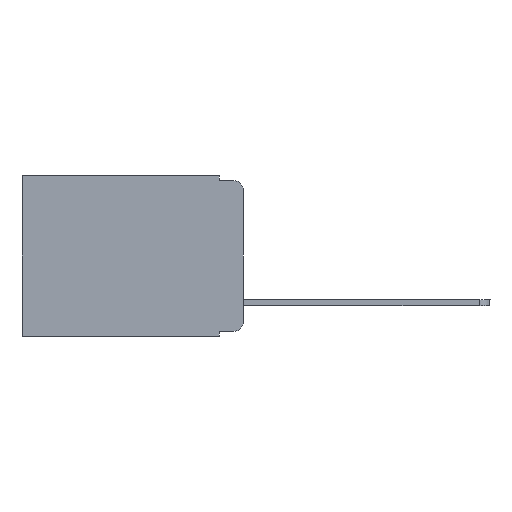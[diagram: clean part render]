
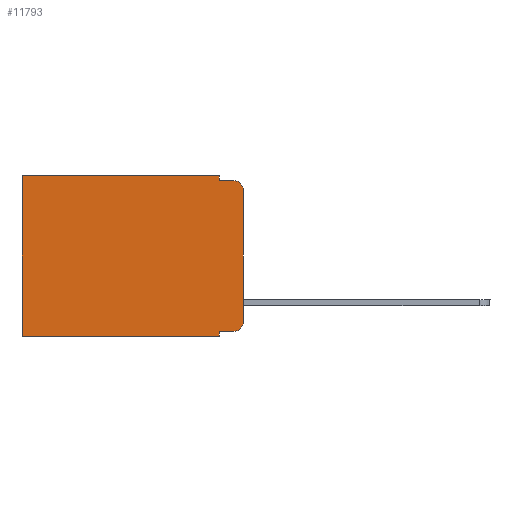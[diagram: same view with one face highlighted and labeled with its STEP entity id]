
A CAD part, left-side view. The second image highlights one B-rep face of the part: STEP entity #11793.
In plain terms, the highlighted planar face has unit normal (-1, 0, 0).
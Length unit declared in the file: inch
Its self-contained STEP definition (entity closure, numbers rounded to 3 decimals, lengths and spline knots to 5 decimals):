
#476 = VERTEX_POINT ( 'NONE', #9377 ) ;
#605 = EDGE_LOOP ( 'NONE', ( #9078, #6765, #993, #13070, #1900, #7192, #5269, #7069, #10858, #4568 ) ) ;
#840 = CARTESIAN_POINT ( 'NONE',  ( 0.298, 0.473, 0. ) ) ;
#993 = ORIENTED_EDGE ( 'NONE', *, *, #6296, .F. ) ;
#1261 = CARTESIAN_POINT ( 'NONE',  ( 0.298, 0.02, -0.03 ) ) ;
#1284 = DIRECTION ( 'NONE',  ( 0., 0., -1. ) ) ;
#1359 = CARTESIAN_POINT ( 'NONE',  ( 0.298, 0.473, -0.343 ) ) ;
#1796 = CARTESIAN_POINT ( 'NONE',  ( 0.298, 0., -0.03 ) ) ;
#1894 = LINE ( 'NONE', #2930, #6676 ) ;
#1900 = ORIENTED_EDGE ( 'NONE', *, *, #7040, .T. ) ;
#1941 = LINE ( 'NONE', #12450, #11049 ) ;
#2186 = PLANE ( 'NONE',  #11965 ) ;
#2492 = VERTEX_POINT ( 'NONE', #10042 ) ;
#2495 = CARTESIAN_POINT ( 'NONE',  ( 0.298, 0.02, -0.333 ) ) ;
#2696 = VECTOR ( 'NONE', #3556, 39.37008 ) ;
#2858 = VERTEX_POINT ( 'NONE', #13397 ) ;
#2930 = CARTESIAN_POINT ( 'NONE',  ( 0.298, 0.051, -0.333 ) ) ;
#3556 = DIRECTION ( 'NONE',  ( 0., 0., -1. ) ) ;
#3610 = DIRECTION ( 'NONE',  ( 0., 1., 0. ) ) ;
#3812 = CARTESIAN_POINT ( 'NONE',  ( 0.298, 0., 0. ) ) ;
#3837 = CARTESIAN_POINT ( 'NONE',  ( 0.298, 0.051, -0.343 ) ) ;
#3900 = DIRECTION ( 'NONE',  ( 0., -1., 0. ) ) ;
#3905 = EDGE_CURVE ( 'NONE', #4209, #2492, #10246, .T. ) ;
#4072 = CIRCLE ( 'NONE', #11988, 0.02 ) ;
#4209 = VERTEX_POINT ( 'NONE', #1796 ) ;
#4471 = DIRECTION ( 'NONE',  ( 1., 0., 0. ) ) ;
#4568 = ORIENTED_EDGE ( 'NONE', *, *, #6722, .T. ) ;
#4793 = CARTESIAN_POINT ( 'NONE',  ( 0.298, 0., -0.313 ) ) ;
#5070 = DIRECTION ( 'NONE',  ( 0., 0., -1. ) ) ;
#5269 = ORIENTED_EDGE ( 'NONE', *, *, #10959, .F. ) ;
#5420 = DIRECTION ( 'NONE',  ( 0., 0., -1. ) ) ;
#5440 = LINE ( 'NONE', #10599, #9110 ) ;
#6147 = VECTOR ( 'NONE', #5070, 39.37008 ) ;
#6296 = EDGE_CURVE ( 'NONE', #476, #2492, #5440, .T. ) ;
#6297 = AXIS2_PLACEMENT_3D ( 'NONE', #1261, #10580, #5420 ) ;
#6389 = DIRECTION ( 'NONE',  ( -1., 0., 0. ) ) ;
#6676 = VECTOR ( 'NONE', #3900, 39.37008 ) ;
#6722 = EDGE_CURVE ( 'NONE', #13594, #12317, #4072, .T. ) ;
#6765 = ORIENTED_EDGE ( 'NONE', *, *, #3905, .T. ) ;
#7040 = EDGE_CURVE ( 'NONE', #8321, #11954, #13282, .T. ) ;
#7058 = EDGE_CURVE ( 'NONE', #11954, #8721, #13421, .T. ) ;
#7069 = ORIENTED_EDGE ( 'NONE', *, *, #11130, .F. ) ;
#7123 = DIRECTION ( 'NONE',  ( 0., 0., -1. ) ) ;
#7192 = ORIENTED_EDGE ( 'NONE', *, *, #7058, .T. ) ;
#7750 = LINE ( 'NONE', #11960, #9729 ) ;
#8321 = VERTEX_POINT ( 'NONE', #10301 ) ;
#8598 = FACE_OUTER_BOUND ( 'NONE', #605, .T. ) ;
#8721 = VERTEX_POINT ( 'NONE', #1359 ) ;
#9078 = ORIENTED_EDGE ( 'NONE', *, *, #11810, .F. ) ;
#9110 = VECTOR ( 'NONE', #11783, 39.37008 ) ;
#9185 = CARTESIAN_POINT ( 'NONE',  ( 0.298, 0.051, 0. ) ) ;
#9193 = DIRECTION ( 'NONE',  ( 0., 1., 0. ) ) ;
#9377 = CARTESIAN_POINT ( 'NONE',  ( 0.298, 0.051, -0.01 ) ) ;
#9729 = VECTOR ( 'NONE', #3610, 39.37008 ) ;
#10042 = CARTESIAN_POINT ( 'NONE',  ( 0.298, 0.02, -0.01 ) ) ;
#10246 = CIRCLE ( 'NONE', #6297, 0.02 ) ;
#10301 = CARTESIAN_POINT ( 'NONE',  ( 0.298, 0.051, 0. ) ) ;
#10580 = DIRECTION ( 'NONE',  ( -1., 0., 0. ) ) ;
#10599 = CARTESIAN_POINT ( 'NONE',  ( 0.298, 0.051, -0.01 ) ) ;
#10739 = CARTESIAN_POINT ( 'NONE',  ( 0.298, 0., 0. ) ) ;
#10858 = ORIENTED_EDGE ( 'NONE', *, *, #12032, .T. ) ;
#10959 = EDGE_CURVE ( 'NONE', #11835, #8721, #7750, .T. ) ;
#11049 = VECTOR ( 'NONE', #7123, 39.37008 ) ;
#11071 = LINE ( 'NONE', #11207, #2696 ) ;
#11130 = EDGE_CURVE ( 'NONE', #2858, #11835, #1941, .T. ) ;
#11207 = CARTESIAN_POINT ( 'NONE',  ( 0.298, 0., 0. ) ) ;
#11245 = DIRECTION ( 'NONE',  ( 0., 0., -1. ) ) ;
#11353 = CARTESIAN_POINT ( 'NONE',  ( 0.298, 0.473, 0. ) ) ;
#11783 = DIRECTION ( 'NONE',  ( 0., -1., 0. ) ) ;
#11793 = ADVANCED_FACE ( 'NONE', ( #8598 ), #2186, .F. ) ;
#11810 = EDGE_CURVE ( 'NONE', #4209, #12317, #11071, .T. ) ;
#11835 = VERTEX_POINT ( 'NONE', #3837 ) ;
#11954 = VERTEX_POINT ( 'NONE', #11353 ) ;
#11960 = CARTESIAN_POINT ( 'NONE',  ( 0.298, 0., -0.343 ) ) ;
#11965 = AXIS2_PLACEMENT_3D ( 'NONE', #10739, #4471, #1284 ) ;
#11988 = AXIS2_PLACEMENT_3D ( 'NONE', #13586, #6389, #13646 ) ;
#12032 = EDGE_CURVE ( 'NONE', #2858, #13594, #1894, .T. ) ;
#12316 = VECTOR ( 'NONE', #9193, 39.37008 ) ;
#12317 = VERTEX_POINT ( 'NONE', #4793 ) ;
#12450 = CARTESIAN_POINT ( 'NONE',  ( 0.298, 0.051, 0. ) ) ;
#12583 = LINE ( 'NONE', #9185, #13532 ) ;
#12631 = EDGE_CURVE ( 'NONE', #8321, #476, #12583, .T. ) ;
#13070 = ORIENTED_EDGE ( 'NONE', *, *, #12631, .F. ) ;
#13282 = LINE ( 'NONE', #3812, #12316 ) ;
#13397 = CARTESIAN_POINT ( 'NONE',  ( 0.298, 0.051, -0.333 ) ) ;
#13421 = LINE ( 'NONE', #840, #6147 ) ;
#13532 = VECTOR ( 'NONE', #11245, 39.37008 ) ;
#13586 = CARTESIAN_POINT ( 'NONE',  ( 0.298, 0.02, -0.313 ) ) ;
#13594 = VERTEX_POINT ( 'NONE', #2495 ) ;
#13646 = DIRECTION ( 'NONE',  ( 0., 0., -1. ) ) ;
